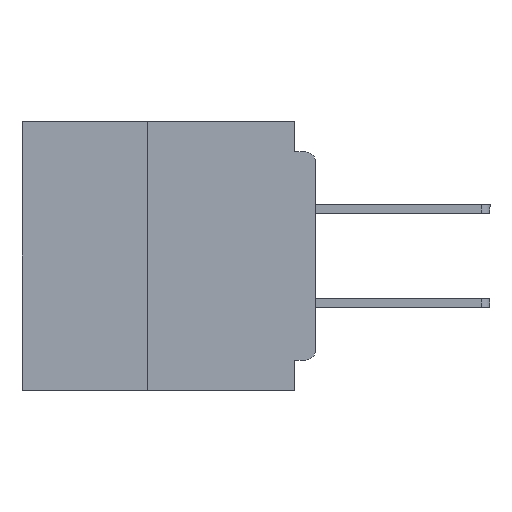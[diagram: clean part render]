
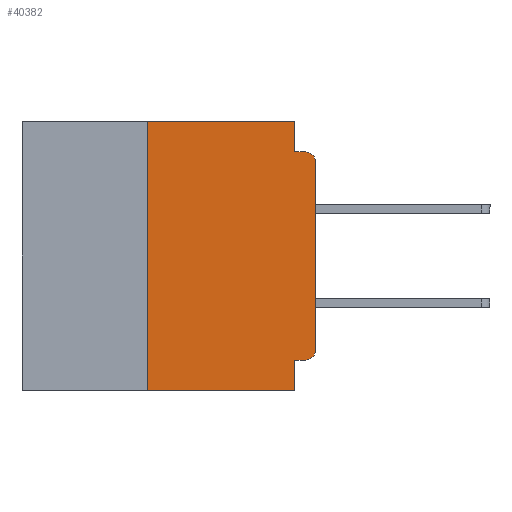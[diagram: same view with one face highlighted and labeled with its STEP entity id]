
A CAD part, left-side view. The second image highlights one B-rep face of the part: STEP entity #40382.
In plain terms, the highlighted planar face has unit normal (-1, 0, 0).
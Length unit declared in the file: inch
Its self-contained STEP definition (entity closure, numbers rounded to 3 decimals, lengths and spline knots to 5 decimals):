
#267 = DIRECTION ( 'NONE',  ( 0., 0., 1. ) ) ;
#2173 = CARTESIAN_POINT ( 'NONE',  ( 0., 0.25, 0. ) ) ;
#4066 = EDGE_CURVE ( 'NONE', #48498, #50737, #11638, .T. ) ;
#4101 = VERTEX_POINT ( 'NONE', #15165 ) ;
#5351 = CARTESIAN_POINT ( 'NONE',  ( 0., 0., -0.06 ) ) ;
#5485 = EDGE_CURVE ( 'NONE', #48498, #8490, #19244, .T. ) ;
#8490 = VERTEX_POINT ( 'NONE', #13600 ) ;
#9769 = ORIENTED_EDGE ( 'NONE', *, *, #5485, .F. ) ;
#10229 = LINE ( 'NONE', #11729, #44774 ) ;
#10683 = EDGE_CURVE ( 'NONE', #23643, #38730, #39984, .T. ) ;
#11133 = DIRECTION ( 'NONE',  ( 0., 0., 1. ) ) ;
#11638 = CIRCLE ( 'NONE', #45783, 0.015 ) ;
#11654 = EDGE_CURVE ( 'NONE', #4101, #19759, #47585, .T. ) ;
#11681 = EDGE_CURVE ( 'NONE', #38730, #55288, #10229, .T. ) ;
#11729 = CARTESIAN_POINT ( 'NONE',  ( 0., 0., -0.045 ) ) ;
#13600 = CARTESIAN_POINT ( 'NONE',  ( 0., 0.031, -0.355 ) ) ;
#13779 = CARTESIAN_POINT ( 'NONE',  ( 0., 0., 0. ) ) ;
#15165 = CARTESIAN_POINT ( 'NONE',  ( 0., 0.25, -0.4 ) ) ;
#16099 = CARTESIAN_POINT ( 'NONE',  ( 0., 0.25, -0.4 ) ) ;
#16305 = DIRECTION ( 'NONE',  ( 0., -1., 0. ) ) ;
#18091 = CARTESIAN_POINT ( 'NONE',  ( 0., 0., -0.34 ) ) ;
#18166 = DIRECTION ( 'NONE',  ( 0., 0., -1. ) ) ;
#18405 = EDGE_CURVE ( 'NONE', #8490, #19600, #49922, .T. ) ;
#18407 = DIRECTION ( 'NONE',  ( 0., 0., -1. ) ) ;
#18460 = DIRECTION ( 'NONE',  ( -1., 0., 0. ) ) ;
#19208 = VECTOR ( 'NONE', #55180, 39.37008 ) ;
#19225 = CARTESIAN_POINT ( 'NONE',  ( 0., 0.015, -0.34 ) ) ;
#19244 = LINE ( 'NONE', #49832, #44633 ) ;
#19600 = VERTEX_POINT ( 'NONE', #41827 ) ;
#19759 = VERTEX_POINT ( 'NONE', #2173 ) ;
#20475 = EDGE_LOOP ( 'NONE', ( #56430, #23897, #33659, #28697, #55716, #35678, #27916, #55189, #9769, #46149 ) ) ;
#21900 = CARTESIAN_POINT ( 'NONE',  ( 0., 0.031, -0.045 ) ) ;
#22775 = VECTOR ( 'NONE', #267, 39.37008 ) ;
#22873 = DIRECTION ( 'NONE',  ( 0., 1., 0. ) ) ;
#23102 = EDGE_CURVE ( 'NONE', #50737, #27526, #57184, .T. ) ;
#23643 = VERTEX_POINT ( 'NONE', #48973 ) ;
#23897 = ORIENTED_EDGE ( 'NONE', *, *, #31922, .T. ) ;
#24352 = CARTESIAN_POINT ( 'NONE',  ( 0., 0.015, -0.06 ) ) ;
#25179 = DIRECTION ( 'NONE',  ( 1., 0., 0. ) ) ;
#25973 = VECTOR ( 'NONE', #46172, 39.37008 ) ;
#26918 = CARTESIAN_POINT ( 'NONE',  ( 0., 0.437, -0.4 ) ) ;
#27526 = VERTEX_POINT ( 'NONE', #5351 ) ;
#27564 = AXIS2_PLACEMENT_3D ( 'NONE', #24352, #55737, #28817 ) ;
#27916 = ORIENTED_EDGE ( 'NONE', *, *, #55125, .T. ) ;
#28697 = ORIENTED_EDGE ( 'NONE', *, *, #10683, .F. ) ;
#28817 = DIRECTION ( 'NONE',  ( 0., 0., -1. ) ) ;
#31408 = DIRECTION ( 'NONE',  ( 0., -1., 0. ) ) ;
#31922 = EDGE_CURVE ( 'NONE', #27526, #55288, #55474, .T. ) ;
#33123 = VECTOR ( 'NONE', #31408, 39.37008 ) ;
#33659 = ORIENTED_EDGE ( 'NONE', *, *, #11681, .F. ) ;
#33968 = PLANE ( 'NONE',  #45295 ) ;
#35678 = ORIENTED_EDGE ( 'NONE', *, *, #11654, .F. ) ;
#36162 = EDGE_CURVE ( 'NONE', #19759, #23643, #55044, .T. ) ;
#38730 = VERTEX_POINT ( 'NONE', #21900 ) ;
#39984 = LINE ( 'NONE', #45151, #42792 ) ;
#40382 = ADVANCED_FACE ( 'NONE', ( #49358 ), #33968, .F. ) ;
#41622 = CARTESIAN_POINT ( 'NONE',  ( 0., 0.031, -0.4 ) ) ;
#41827 = CARTESIAN_POINT ( 'NONE',  ( 0., 0.031, -0.4 ) ) ;
#41950 = CARTESIAN_POINT ( 'NONE',  ( 0., 0.015, -0.355 ) ) ;
#42792 = VECTOR ( 'NONE', #18166, 39.37008 ) ;
#44633 = VECTOR ( 'NONE', #22873, 39.37008 ) ;
#44774 = VECTOR ( 'NONE', #16305, 39.37008 ) ;
#45151 = CARTESIAN_POINT ( 'NONE',  ( 0., 0.031, 0. ) ) ;
#45295 = AXIS2_PLACEMENT_3D ( 'NONE', #52116, #25179, #56569 ) ;
#45783 = AXIS2_PLACEMENT_3D ( 'NONE', #19225, #18460, #18407 ) ;
#46149 = ORIENTED_EDGE ( 'NONE', *, *, #4066, .T. ) ;
#46172 = DIRECTION ( 'NONE',  ( 0., 0., -1. ) ) ;
#47585 = LINE ( 'NONE', #16099, #56625 ) ;
#48498 = VERTEX_POINT ( 'NONE', #41950 ) ;
#48973 = CARTESIAN_POINT ( 'NONE',  ( 0., 0.031, 0. ) ) ;
#49358 = FACE_OUTER_BOUND ( 'NONE', #20475, .T. ) ;
#49832 = CARTESIAN_POINT ( 'NONE',  ( 0., 0., -0.355 ) ) ;
#49922 = LINE ( 'NONE', #41622, #25973 ) ;
#50341 = CARTESIAN_POINT ( 'NONE',  ( 0., 0.015, -0.045 ) ) ;
#50727 = CARTESIAN_POINT ( 'NONE',  ( 0., 0.437, 0. ) ) ;
#50737 = VERTEX_POINT ( 'NONE', #18091 ) ;
#52116 = CARTESIAN_POINT ( 'NONE',  ( 0., 0.437, 0. ) ) ;
#55044 = LINE ( 'NONE', #50727, #19208 ) ;
#55125 = EDGE_CURVE ( 'NONE', #4101, #19600, #57659, .T. ) ;
#55180 = DIRECTION ( 'NONE',  ( 0., -1., 0. ) ) ;
#55189 = ORIENTED_EDGE ( 'NONE', *, *, #18405, .F. ) ;
#55288 = VERTEX_POINT ( 'NONE', #50341 ) ;
#55474 = CIRCLE ( 'NONE', #27564, 0.015 ) ;
#55716 = ORIENTED_EDGE ( 'NONE', *, *, #36162, .F. ) ;
#55737 = DIRECTION ( 'NONE',  ( -1., 0., 0. ) ) ;
#56430 = ORIENTED_EDGE ( 'NONE', *, *, #23102, .T. ) ;
#56569 = DIRECTION ( 'NONE',  ( 0., 0., -1. ) ) ;
#56625 = VECTOR ( 'NONE', #11133, 39.37008 ) ;
#57184 = LINE ( 'NONE', #13779, #22775 ) ;
#57659 = LINE ( 'NONE', #26918, #33123 ) ;
